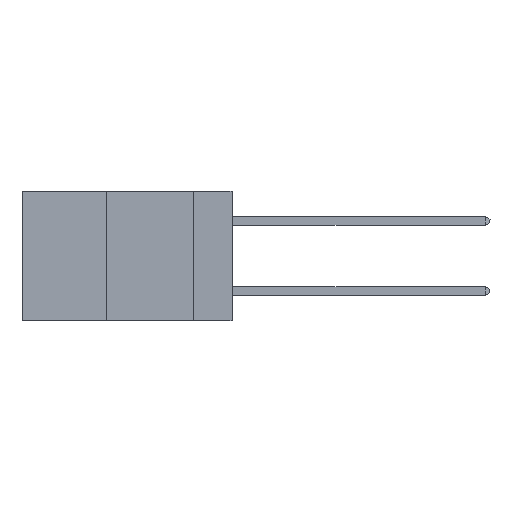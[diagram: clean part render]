
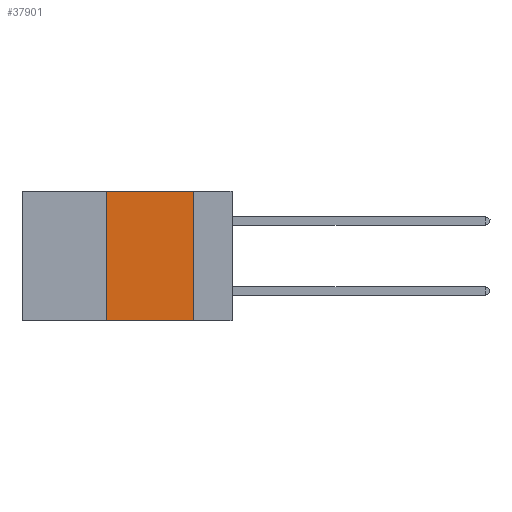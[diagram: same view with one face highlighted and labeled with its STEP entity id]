
A CAD part, left-side view. The second image highlights one B-rep face of the part: STEP entity #37901.
In plain terms, the highlighted planar face has unit normal (-1, 0, 0).
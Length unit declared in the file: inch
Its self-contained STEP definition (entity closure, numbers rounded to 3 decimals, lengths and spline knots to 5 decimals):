
#290 = ORIENTED_EDGE ( 'NONE', *, *, #30123, .T. ) ;
#409 = DIRECTION ( 'NONE',  ( 0., 0., -1. ) ) ;
#1207 = VECTOR ( 'NONE', #35614, 39.37008 ) ;
#2049 = DIRECTION ( 'NONE',  ( 0., -1., 0. ) ) ;
#3182 = ORIENTED_EDGE ( 'NONE', *, *, #3190, .F. ) ;
#3190 = EDGE_CURVE ( 'NONE', #39078, #22815, #37811, .T. ) ;
#3796 = CARTESIAN_POINT ( 'NONE',  ( 0., 0.11, 0. ) ) ;
#4979 = CARTESIAN_POINT ( 'NONE',  ( 0., 0.11, 0. ) ) ;
#7133 = CARTESIAN_POINT ( 'NONE',  ( 0., 0.6, 0. ) ) ;
#9606 = ORIENTED_EDGE ( 'NONE', *, *, #45402, .F. ) ;
#13709 = CARTESIAN_POINT ( 'NONE',  ( 0., 0.36, 0. ) ) ;
#15104 = LINE ( 'NONE', #7133, #1207 ) ;
#16859 = DIRECTION ( 'NONE',  ( 0., 0., 1. ) ) ;
#17881 = VECTOR ( 'NONE', #2049, 39.37008 ) ;
#21094 = CARTESIAN_POINT ( 'NONE',  ( 0., 0.36, 0. ) ) ;
#22815 = VERTEX_POINT ( 'NONE', #45889 ) ;
#24702 = EDGE_LOOP ( 'NONE', ( #3182, #9606, #30122, #290 ) ) ;
#25098 = PLANE ( 'NONE',  #29583 ) ;
#26160 = LINE ( 'NONE', #41405, #17881 ) ;
#26694 = EDGE_CURVE ( 'NONE', #33717, #43971, #33694, .T. ) ;
#28967 = CARTESIAN_POINT ( 'NONE',  ( 0., 0.6, 0. ) ) ;
#29486 = VECTOR ( 'NONE', #29765, 39.37008 ) ;
#29583 = AXIS2_PLACEMENT_3D ( 'NONE', #28967, #42711, #409 ) ;
#29765 = DIRECTION ( 'NONE',  ( 0., 0., -1. ) ) ;
#30122 = ORIENTED_EDGE ( 'NONE', *, *, #26694, .F. ) ;
#30123 = EDGE_CURVE ( 'NONE', #33717, #22815, #26160, .T. ) ;
#30248 = FACE_OUTER_BOUND ( 'NONE', #24702, .T. ) ;
#30925 = VECTOR ( 'NONE', #16859, 39.37008 ) ;
#31930 = CARTESIAN_POINT ( 'NONE',  ( 0., 0.36, -0.37 ) ) ;
#33694 = LINE ( 'NONE', #13709, #30925 ) ;
#33717 = VERTEX_POINT ( 'NONE', #31930 ) ;
#35614 = DIRECTION ( 'NONE',  ( 0., -1., 0. ) ) ;
#37811 = LINE ( 'NONE', #4979, #29486 ) ;
#37901 = ADVANCED_FACE ( 'NONE', ( #30248 ), #25098, .F. ) ;
#39078 = VERTEX_POINT ( 'NONE', #3796 ) ;
#41405 = CARTESIAN_POINT ( 'NONE',  ( 0., 0.6, -0.37 ) ) ;
#42711 = DIRECTION ( 'NONE',  ( 1., 0., 0. ) ) ;
#43971 = VERTEX_POINT ( 'NONE', #21094 ) ;
#45402 = EDGE_CURVE ( 'NONE', #43971, #39078, #15104, .T. ) ;
#45889 = CARTESIAN_POINT ( 'NONE',  ( 0., 0.11, -0.37 ) ) ;
